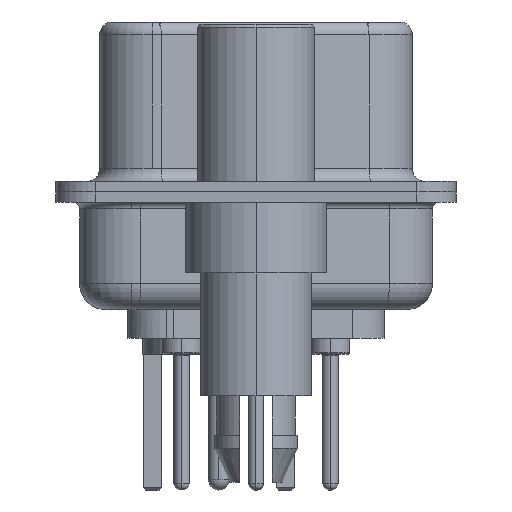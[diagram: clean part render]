
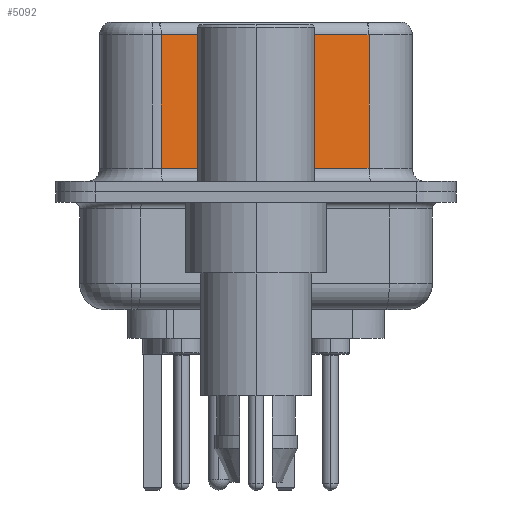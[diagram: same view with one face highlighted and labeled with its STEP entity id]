
A CAD part, left-side view. The second image highlights one B-rep face of the part: STEP entity #5092.
In plain terms, the highlighted planar face has unit normal (-0.985, -0.174, 0).
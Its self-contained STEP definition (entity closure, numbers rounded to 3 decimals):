
#639 = VECTOR ( 'NONE', #28558, 1000. ) ;
#1285 = AXIS2_PLACEMENT_3D ( 'NONE', #6963, #14000, #6794 ) ;
#1908 = EDGE_CURVE ( 'NONE', #17606, #8876, #22076, .T. ) ;
#3215 = CARTESIAN_POINT ( 'NONE',  ( 5.132, -4.322, 0.9 ) ) ;
#3883 = LINE ( 'NONE', #12366, #10061 ) ;
#5092 = ADVANCED_FACE ( 'NONE', ( #9179 ), #15704, .F. ) ;
#6078 = LINE ( 'NONE', #27535, #33525 ) ;
#6794 = DIRECTION ( 'NONE',  ( -0.174, 0.985, 0. ) ) ;
#6963 = CARTESIAN_POINT ( 'NONE',  ( 5.132, -4.322, 6.52 ) ) ;
#7707 = LINE ( 'NONE', #20484, #639 ) ;
#8876 = VERTEX_POINT ( 'NONE', #14179 ) ;
#9179 = FACE_OUTER_BOUND ( 'NONE', #28045, .T. ) ;
#9597 = VECTOR ( 'NONE', #11333, 1000. ) ;
#10061 = VECTOR ( 'NONE', #30965, 1000. ) ;
#10062 = CARTESIAN_POINT ( 'NONE',  ( 3.73, 3.628, 6.02 ) ) ;
#10766 = EDGE_CURVE ( 'NONE', #18557, #8876, #3883, .T. ) ;
#11075 = ORIENTED_EDGE ( 'NONE', *, *, #10766, .F. ) ;
#11252 = ORIENTED_EDGE ( 'NONE', *, *, #23956, .T. ) ;
#11333 = DIRECTION ( 'NONE',  ( 0.174, -0.985, 0. ) ) ;
#12366 = CARTESIAN_POINT ( 'NONE',  ( 5.132, -4.322, 6.52 ) ) ;
#14000 = DIRECTION ( 'NONE',  ( 0.985, 0.174, 0. ) ) ;
#14179 = CARTESIAN_POINT ( 'NONE',  ( 5.132, -4.322, 0.9 ) ) ;
#15704 = PLANE ( 'NONE',  #1285 ) ;
#16726 = CARTESIAN_POINT ( 'NONE',  ( 5.132, -4.322, 6.02 ) ) ;
#17606 = VERTEX_POINT ( 'NONE', #31728 ) ;
#18162 = EDGE_CURVE ( 'NONE', #18557, #28670, #7707, .T. ) ;
#18557 = VERTEX_POINT ( 'NONE', #16726 ) ;
#19150 = ORIENTED_EDGE ( 'NONE', *, *, #1908, .T. ) ;
#19160 = ORIENTED_EDGE ( 'NONE', *, *, #18162, .T. ) ;
#20484 = CARTESIAN_POINT ( 'NONE',  ( 5.132, -4.322, 6.02 ) ) ;
#22076 = LINE ( 'NONE', #3215, #9597 ) ;
#23956 = EDGE_CURVE ( 'NONE', #28670, #17606, #6078, .T. ) ;
#27535 = CARTESIAN_POINT ( 'NONE',  ( 3.73, 3.628, 6.52 ) ) ;
#28045 = EDGE_LOOP ( 'NONE', ( #11075, #19160, #11252, #19150 ) ) ;
#28558 = DIRECTION ( 'NONE',  ( -0.174, 0.985, 0. ) ) ;
#28670 = VERTEX_POINT ( 'NONE', #10062 ) ;
#30965 = DIRECTION ( 'NONE',  ( 0., 0., -1. ) ) ;
#31728 = CARTESIAN_POINT ( 'NONE',  ( 3.73, 3.628, 0.9 ) ) ;
#32902 = DIRECTION ( 'NONE',  ( 0., 0., -1. ) ) ;
#33525 = VECTOR ( 'NONE', #32902, 1000. ) ;
